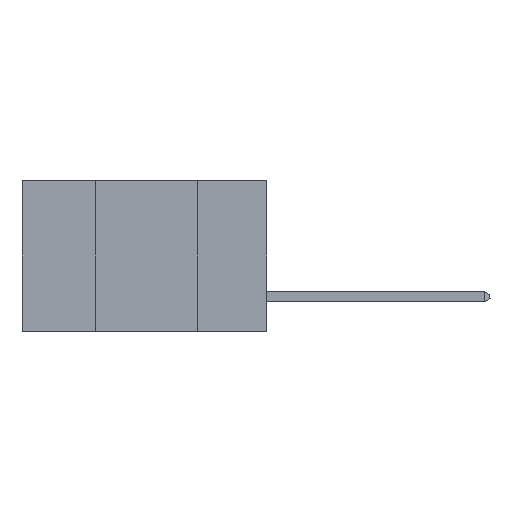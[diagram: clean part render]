
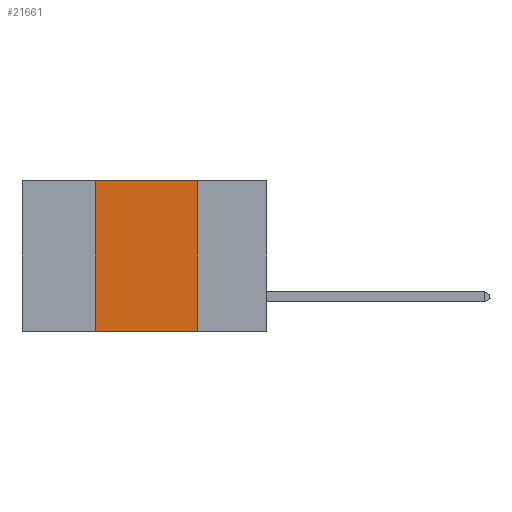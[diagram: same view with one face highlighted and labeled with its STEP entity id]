
A CAD part, left-side view. The second image highlights one B-rep face of the part: STEP entity #21661.
In plain terms, the highlighted planar face has unit normal (-1, 0, 0).
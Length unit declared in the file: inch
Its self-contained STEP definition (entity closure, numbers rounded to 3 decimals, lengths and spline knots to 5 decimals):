
#434 = EDGE_CURVE ( 'NONE', #15774, #12581, #1430, .T. ) ;
#1430 = LINE ( 'NONE', #23939, #8865 ) ;
#1765 = EDGE_CURVE ( 'NONE', #15774, #9747, #21490, .T. ) ;
#2746 = AXIS2_PLACEMENT_3D ( 'NONE', #23021, #7365, #21249 ) ;
#3282 = LINE ( 'NONE', #18594, #15993 ) ;
#4457 = LINE ( 'NONE', #5779, #19032 ) ;
#5779 = CARTESIAN_POINT ( 'NONE',  ( 0., 0.17, 0. ) ) ;
#5791 = CARTESIAN_POINT ( 'NONE',  ( 0., 0.42, -0.37 ) ) ;
#6708 = DIRECTION ( 'NONE',  ( 0., -1., 0. ) ) ;
#6845 = VERTEX_POINT ( 'NONE', #11488 ) ;
#7365 = DIRECTION ( 'NONE',  ( 1., 0., 0. ) ) ;
#7808 = EDGE_CURVE ( 'NONE', #6845, #9747, #4457, .T. ) ;
#8865 = VECTOR ( 'NONE', #20293, 39.37008 ) ;
#9199 = PLANE ( 'NONE',  #2746 ) ;
#9747 = VERTEX_POINT ( 'NONE', #10637 ) ;
#10637 = CARTESIAN_POINT ( 'NONE',  ( 0., 0.17, -0.37 ) ) ;
#11488 = CARTESIAN_POINT ( 'NONE',  ( 0., 0.17, 0. ) ) ;
#12581 = VERTEX_POINT ( 'NONE', #15730 ) ;
#15630 = CARTESIAN_POINT ( 'NONE',  ( 0., 0.6, -0.37 ) ) ;
#15730 = CARTESIAN_POINT ( 'NONE',  ( 0., 0.42, 0. ) ) ;
#15774 = VERTEX_POINT ( 'NONE', #5791 ) ;
#15792 = ORIENTED_EDGE ( 'NONE', *, *, #1765, .T. ) ;
#15993 = VECTOR ( 'NONE', #6708, 39.37008 ) ;
#16196 = VECTOR ( 'NONE', #17727, 39.37008 ) ;
#17582 = FACE_OUTER_BOUND ( 'NONE', #24357, .T. ) ;
#17727 = DIRECTION ( 'NONE',  ( 0., -1., 0. ) ) ;
#18594 = CARTESIAN_POINT ( 'NONE',  ( 0., 0.6, 0. ) ) ;
#19032 = VECTOR ( 'NONE', #23739, 39.37008 ) ;
#20293 = DIRECTION ( 'NONE',  ( 0., 0., 1. ) ) ;
#20513 = ORIENTED_EDGE ( 'NONE', *, *, #21042, .F. ) ;
#21042 = EDGE_CURVE ( 'NONE', #12581, #6845, #3282, .T. ) ;
#21249 = DIRECTION ( 'NONE',  ( 0., 0., -1. ) ) ;
#21490 = LINE ( 'NONE', #15630, #16196 ) ;
#21661 = ADVANCED_FACE ( 'NONE', ( #17582 ), #9199, .F. ) ;
#21739 = ORIENTED_EDGE ( 'NONE', *, *, #434, .F. ) ;
#23021 = CARTESIAN_POINT ( 'NONE',  ( 0., 0.6, 0. ) ) ;
#23739 = DIRECTION ( 'NONE',  ( 0., 0., -1. ) ) ;
#23939 = CARTESIAN_POINT ( 'NONE',  ( 0., 0.42, 0. ) ) ;
#24357 = EDGE_LOOP ( 'NONE', ( #24606, #20513, #21739, #15792 ) ) ;
#24606 = ORIENTED_EDGE ( 'NONE', *, *, #7808, .F. ) ;
